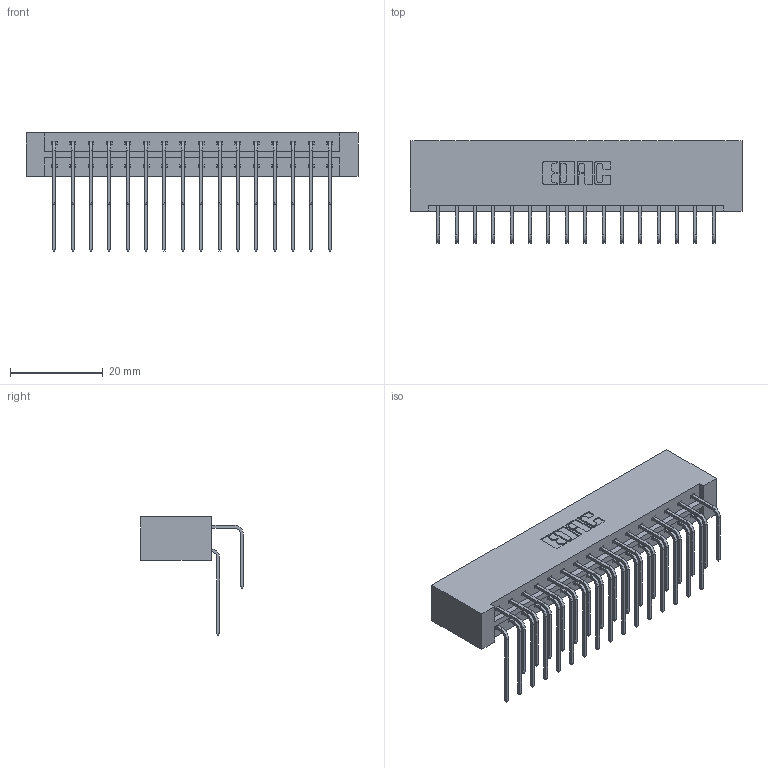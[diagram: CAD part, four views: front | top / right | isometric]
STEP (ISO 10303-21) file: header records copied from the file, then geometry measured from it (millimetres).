
FILE_DESCRIPTION (( 'STEP AP203' ), '1' );
FILE_NAME ('833-032-558-201.STEP', '2020-06-02T19:03:45', ( '' ), ( '' ), 'SwSTEP 2.0', 'SolidWorks 2020', '' );
FILE_SCHEMA (( 'CONFIG_CONTROL_DESIGN' ));
Length unit declared in the file: inch
Products named in the file (4): 345-292-001_558 Tail - 2; 833-032-558-201; 833 Part_Lugless; 345-292-001_558 559 Tail - 1
Assembly tree (33 placements, depth 2):
  833-032-558-201
    833 Part_Lugless
    345-292-001_558 559 Tail - 1  x16
    345-292-001_558 Tail - 2  x16
Bounding box: 71.65 x 22.17 x 25.53 mm (x, y, z)
Volume: 7889.1 mm3; surface area: 9991.3 mm2
Topology: 33 solids, 33 shells, 1834 faces, 5439 edges, 3582 vertices
Faces by surface type: plane 1282, cylinder 552
Entity records: 15163 total; most frequent: CARTESIAN_POINT 2593, ORIENTED_EDGE 2478, DIRECTION 2235, EDGE_CURVE 1239, LINE 1079, VECTOR 1079, VERTEX_POINT 822, AXIS2_PLACEMENT_3D 578
